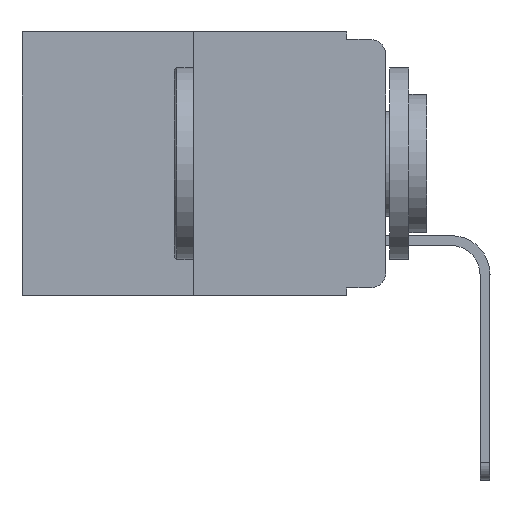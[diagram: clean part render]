
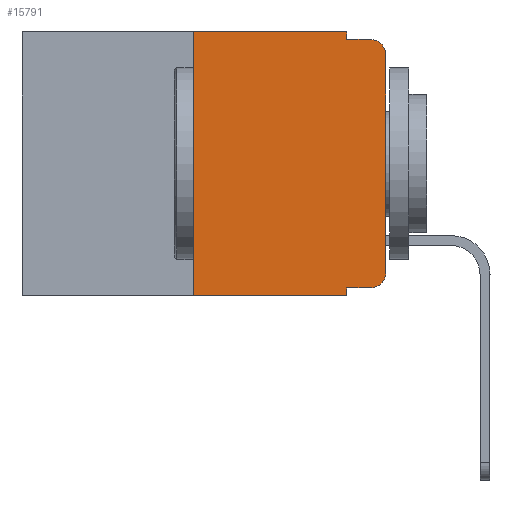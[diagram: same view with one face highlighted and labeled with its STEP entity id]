
A CAD part, left-side view. The second image highlights one B-rep face of the part: STEP entity #15791.
In plain terms, the highlighted planar face has unit normal (-1, 0, 0).
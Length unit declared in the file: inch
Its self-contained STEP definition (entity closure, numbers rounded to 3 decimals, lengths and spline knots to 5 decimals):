
#354 = VERTEX_POINT ( 'NONE', #1058 ) ;
#603 = DIRECTION ( 'NONE',  ( 0., 0., -1. ) ) ;
#785 = CARTESIAN_POINT ( 'NONE',  ( 0., 0., 0. ) ) ;
#793 = CARTESIAN_POINT ( 'NONE',  ( 0., 0.473, -0.343 ) ) ;
#843 = EDGE_CURVE ( 'NONE', #4596, #9434, #10415, .T. ) ;
#953 = DIRECTION ( 'NONE',  ( 0., 0., 1. ) ) ;
#1049 = FACE_OUTER_BOUND ( 'NONE', #5162, .T. ) ;
#1058 = CARTESIAN_POINT ( 'NONE',  ( 0., 0.25, 0. ) ) ;
#1060 = CARTESIAN_POINT ( 'NONE',  ( 0., 0.02, -0.03 ) ) ;
#1208 = CARTESIAN_POINT ( 'NONE',  ( 0., 0.051, 0. ) ) ;
#1616 = CARTESIAN_POINT ( 'NONE',  ( 0., 0.051, 0. ) ) ;
#2098 = DIRECTION ( 'NONE',  ( 0., -1., 0. ) ) ;
#2239 = ORIENTED_EDGE ( 'NONE', *, *, #11273, .T. ) ;
#2523 = VECTOR ( 'NONE', #9219, 39.37008 ) ;
#2651 = CARTESIAN_POINT ( 'NONE',  ( 0., 0., -0.313 ) ) ;
#2781 = CARTESIAN_POINT ( 'NONE',  ( 0., 0.02, -0.01 ) ) ;
#2832 = CARTESIAN_POINT ( 'NONE',  ( 0., 0.473, 0. ) ) ;
#2941 = EDGE_CURVE ( 'NONE', #5456, #4596, #10767, .T. ) ;
#3150 = CARTESIAN_POINT ( 'NONE',  ( 0., 0.02, -0.313 ) ) ;
#3445 = DIRECTION ( 'NONE',  ( 0., 0., 1. ) ) ;
#3795 = ORIENTED_EDGE ( 'NONE', *, *, #6293, .F. ) ;
#4325 = CARTESIAN_POINT ( 'NONE',  ( 0., 0.051, -0.333 ) ) ;
#4596 = VERTEX_POINT ( 'NONE', #8694 ) ;
#4668 = LINE ( 'NONE', #15320, #11087 ) ;
#4883 = CIRCLE ( 'NONE', #5665, 0.02 ) ;
#4920 = ORIENTED_EDGE ( 'NONE', *, *, #14510, .F. ) ;
#5130 = CARTESIAN_POINT ( 'NONE',  ( 0., 0.25, -0.343 ) ) ;
#5162 = EDGE_LOOP ( 'NONE', ( #13603, #12254, #3795, #14494, #11326, #4920, #2239, #12902, #14365, #16607 ) ) ;
#5456 = VERTEX_POINT ( 'NONE', #2651 ) ;
#5609 = VERTEX_POINT ( 'NONE', #1616 ) ;
#5665 = AXIS2_PLACEMENT_3D ( 'NONE', #3150, #15789, #12091 ) ;
#6112 = DIRECTION ( 'NONE',  ( 0., -1., 0. ) ) ;
#6293 = EDGE_CURVE ( 'NONE', #7466, #9434, #9628, .T. ) ;
#6302 = DIRECTION ( 'NONE',  ( 0., 0., -1. ) ) ;
#6488 = CARTESIAN_POINT ( 'NONE',  ( 0., 0.051, -0.01 ) ) ;
#6652 = VERTEX_POINT ( 'NONE', #4325 ) ;
#6709 = LINE ( 'NONE', #11315, #16517 ) ;
#7131 = CARTESIAN_POINT ( 'NONE',  ( 0., 0.473, 0. ) ) ;
#7352 = VECTOR ( 'NONE', #953, 39.37008 ) ;
#7466 = VERTEX_POINT ( 'NONE', #6488 ) ;
#7654 = DIRECTION ( 'NONE',  ( 0., 0., -1. ) ) ;
#8580 = AXIS2_PLACEMENT_3D ( 'NONE', #7131, #12249, #603 ) ;
#8597 = EDGE_CURVE ( 'NONE', #6652, #11498, #6709, .T. ) ;
#8685 = CARTESIAN_POINT ( 'NONE',  ( 0., 0.25, 0. ) ) ;
#8694 = CARTESIAN_POINT ( 'NONE',  ( 0., 0., -0.03 ) ) ;
#9034 = VECTOR ( 'NONE', #9458, 39.37008 ) ;
#9219 = DIRECTION ( 'NONE',  ( 0., -1., 0. ) ) ;
#9434 = VERTEX_POINT ( 'NONE', #2781 ) ;
#9458 = DIRECTION ( 'NONE',  ( 0., -1., 0. ) ) ;
#9557 = LINE ( 'NONE', #8685, #7352 ) ;
#9628 = LINE ( 'NONE', #10755, #9034 ) ;
#9696 = CARTESIAN_POINT ( 'NONE',  ( 0., 0.051, -0.343 ) ) ;
#10149 = LINE ( 'NONE', #2832, #2523 ) ;
#10345 = AXIS2_PLACEMENT_3D ( 'NONE', #1060, #15305, #6302 ) ;
#10415 = CIRCLE ( 'NONE', #10345, 0.02 ) ;
#10755 = CARTESIAN_POINT ( 'NONE',  ( 0., 0.051, -0.01 ) ) ;
#10767 = LINE ( 'NONE', #785, #15354 ) ;
#11087 = VECTOR ( 'NONE', #7654, 39.37008 ) ;
#11273 = EDGE_CURVE ( 'NONE', #14028, #16399, #13035, .T. ) ;
#11315 = CARTESIAN_POINT ( 'NONE',  ( 0., 0.051, -0.333 ) ) ;
#11326 = ORIENTED_EDGE ( 'NONE', *, *, #14795, .F. ) ;
#11443 = VECTOR ( 'NONE', #2098, 39.37008 ) ;
#11498 = VERTEX_POINT ( 'NONE', #11776 ) ;
#11639 = DIRECTION ( 'NONE',  ( 0., 0., -1. ) ) ;
#11776 = CARTESIAN_POINT ( 'NONE',  ( 0., 0.02, -0.333 ) ) ;
#11891 = VECTOR ( 'NONE', #11639, 39.37008 ) ;
#12091 = DIRECTION ( 'NONE',  ( 0., 0., -1. ) ) ;
#12201 = PLANE ( 'NONE',  #8580 ) ;
#12249 = DIRECTION ( 'NONE',  ( 1., 0., 0. ) ) ;
#12254 = ORIENTED_EDGE ( 'NONE', *, *, #843, .T. ) ;
#12902 = ORIENTED_EDGE ( 'NONE', *, *, #15310, .F. ) ;
#13035 = LINE ( 'NONE', #793, #11443 ) ;
#13603 = ORIENTED_EDGE ( 'NONE', *, *, #2941, .T. ) ;
#14028 = VERTEX_POINT ( 'NONE', #5130 ) ;
#14365 = ORIENTED_EDGE ( 'NONE', *, *, #8597, .T. ) ;
#14494 = ORIENTED_EDGE ( 'NONE', *, *, #16571, .F. ) ;
#14510 = EDGE_CURVE ( 'NONE', #14028, #354, #9557, .T. ) ;
#14795 = EDGE_CURVE ( 'NONE', #354, #5609, #10149, .T. ) ;
#15305 = DIRECTION ( 'NONE',  ( -1., 0., 0. ) ) ;
#15307 = LINE ( 'NONE', #1208, #11891 ) ;
#15310 = EDGE_CURVE ( 'NONE', #6652, #16399, #15307, .T. ) ;
#15320 = CARTESIAN_POINT ( 'NONE',  ( 0., 0.051, 0. ) ) ;
#15354 = VECTOR ( 'NONE', #3445, 39.37008 ) ;
#15746 = EDGE_CURVE ( 'NONE', #11498, #5456, #4883, .T. ) ;
#15789 = DIRECTION ( 'NONE',  ( -1., 0., 0. ) ) ;
#15791 = ADVANCED_FACE ( 'NONE', ( #1049 ), #12201, .F. ) ;
#16399 = VERTEX_POINT ( 'NONE', #9696 ) ;
#16517 = VECTOR ( 'NONE', #6112, 39.37008 ) ;
#16571 = EDGE_CURVE ( 'NONE', #5609, #7466, #4668, .T. ) ;
#16607 = ORIENTED_EDGE ( 'NONE', *, *, #15746, .T. ) ;
